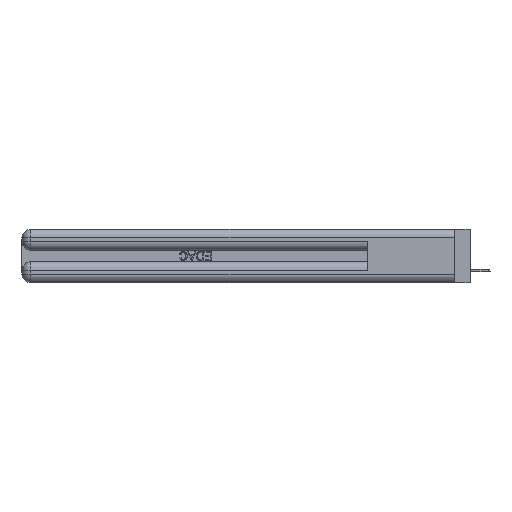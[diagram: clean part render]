
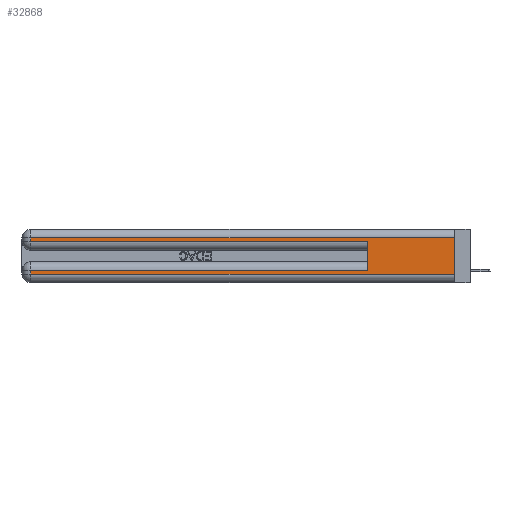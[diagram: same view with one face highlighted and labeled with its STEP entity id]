
A CAD part, left-side view. The second image highlights one B-rep face of the part: STEP entity #32868.
In plain terms, the highlighted planar face has unit normal (-1, 0, 0).
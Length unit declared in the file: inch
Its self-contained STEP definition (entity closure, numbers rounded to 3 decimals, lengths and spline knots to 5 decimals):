
#150 = LINE ( 'NONE', #11200, #28709 ) ;
#1371 = DIRECTION ( 'NONE',  ( 0., 0., -1. ) ) ;
#2030 = VECTOR ( 'NONE', #20193, 39.37008 ) ;
#3878 = VERTEX_POINT ( 'NONE', #27649 ) ;
#4669 = LINE ( 'NONE', #41682, #38491 ) ;
#5585 = LINE ( 'NONE', #27483, #32749 ) ;
#6645 = LINE ( 'NONE', #21100, #47113 ) ;
#8307 = DIRECTION ( 'NONE',  ( 0., 0., -1. ) ) ;
#8576 = PLANE ( 'NONE',  #41972 ) ;
#8738 = DIRECTION ( 'NONE',  ( 0., 0., -1. ) ) ;
#9347 = LINE ( 'NONE', #41319, #2030 ) ;
#10031 = EDGE_CURVE ( 'NONE', #31269, #13768, #5585, .T. ) ;
#10715 = VECTOR ( 'NONE', #8738, 39.37008 ) ;
#11078 = EDGE_CURVE ( 'NONE', #11703, #34523, #15241, .T. ) ;
#11200 = CARTESIAN_POINT ( 'NONE',  ( 0., 2.94, 0.37 ) ) ;
#11703 = VERTEX_POINT ( 'NONE', #31270 ) ;
#12193 = FACE_OUTER_BOUND ( 'NONE', #21809, .T. ) ;
#13702 = DIRECTION ( 'NONE',  ( 0., -1., 0. ) ) ;
#13768 = VERTEX_POINT ( 'NONE', #15794 ) ;
#15241 = LINE ( 'NONE', #32609, #22085 ) ;
#15722 = DIRECTION ( 'NONE',  ( 0., 1., 0. ) ) ;
#15794 = CARTESIAN_POINT ( 'NONE',  ( 0., 2.94, 0.06 ) ) ;
#15911 = ORIENTED_EDGE ( 'NONE', *, *, #23854, .T. ) ;
#17156 = ORIENTED_EDGE ( 'NONE', *, *, #30533, .F. ) ;
#18397 = EDGE_CURVE ( 'NONE', #34523, #3878, #150, .T. ) ;
#19479 = ORIENTED_EDGE ( 'NONE', *, *, #11078, .T. ) ;
#19950 = EDGE_CURVE ( 'NONE', #3878, #29705, #6645, .T. ) ;
#19963 = ORIENTED_EDGE ( 'NONE', *, *, #18397, .T. ) ;
#20193 = DIRECTION ( 'NONE',  ( 0., 1., 0. ) ) ;
#21100 = CARTESIAN_POINT ( 'NONE',  ( 0., 0., 0.285 ) ) ;
#21809 = EDGE_LOOP ( 'NONE', ( #17156, #19479, #19963, #46798, #38950, #22909, #43696, #15911 ) ) ;
#22085 = VECTOR ( 'NONE', #15722, 39.37008 ) ;
#22909 = ORIENTED_EDGE ( 'NONE', *, *, #34354, .T. ) ;
#23854 = EDGE_CURVE ( 'NONE', #13768, #40023, #25228, .T. ) ;
#25228 = LINE ( 'NONE', #28838, #31165 ) ;
#26618 = DIRECTION ( 'NONE',  ( 1., 0., 0. ) ) ;
#27032 = LINE ( 'NONE', #41670, #10715 ) ;
#27483 = CARTESIAN_POINT ( 'NONE',  ( 0., 2.94, 0.37 ) ) ;
#27649 = CARTESIAN_POINT ( 'NONE',  ( 0., 2.94, 0.285 ) ) ;
#28068 = DIRECTION ( 'NONE',  ( 0., -1., 0. ) ) ;
#28709 = VECTOR ( 'NONE', #8307, 39.37008 ) ;
#28838 = CARTESIAN_POINT ( 'NONE',  ( 0., 0., 0.06 ) ) ;
#29705 = VERTEX_POINT ( 'NONE', #42222 ) ;
#30533 = EDGE_CURVE ( 'NONE', #11703, #40023, #27032, .T. ) ;
#30535 = CARTESIAN_POINT ( 'NONE',  ( 0., 0.6, 0.085 ) ) ;
#31165 = VECTOR ( 'NONE', #13702, 39.37008 ) ;
#31269 = VERTEX_POINT ( 'NONE', #40127 ) ;
#31270 = CARTESIAN_POINT ( 'NONE',  ( 0., 0., 0.31 ) ) ;
#32609 = CARTESIAN_POINT ( 'NONE',  ( 0., 0., 0.31 ) ) ;
#32749 = VECTOR ( 'NONE', #42121, 39.37008 ) ;
#32868 = ADVANCED_FACE ( 'NONE', ( #12193 ), #8576, .F. ) ;
#34354 = EDGE_CURVE ( 'NONE', #35734, #31269, #9347, .T. ) ;
#34523 = VERTEX_POINT ( 'NONE', #38905 ) ;
#35734 = VERTEX_POINT ( 'NONE', #30535 ) ;
#37898 = CARTESIAN_POINT ( 'NONE',  ( 0., 0., 0.37 ) ) ;
#38073 = DIRECTION ( 'NONE',  ( 0., 0., 1. ) ) ;
#38491 = VECTOR ( 'NONE', #38073, 39.37008 ) ;
#38905 = CARTESIAN_POINT ( 'NONE',  ( 0., 2.94, 0.31 ) ) ;
#38950 = ORIENTED_EDGE ( 'NONE', *, *, #41998, .F. ) ;
#40023 = VERTEX_POINT ( 'NONE', #44696 ) ;
#40127 = CARTESIAN_POINT ( 'NONE',  ( 0., 2.94, 0.085 ) ) ;
#41319 = CARTESIAN_POINT ( 'NONE',  ( 0., 0., 0.085 ) ) ;
#41670 = CARTESIAN_POINT ( 'NONE',  ( 0., 0., 0.37 ) ) ;
#41682 = CARTESIAN_POINT ( 'NONE',  ( 0., 0.6, 0.145 ) ) ;
#41972 = AXIS2_PLACEMENT_3D ( 'NONE', #37898, #26618, #1371 ) ;
#41998 = EDGE_CURVE ( 'NONE', #35734, #29705, #4669, .T. ) ;
#42121 = DIRECTION ( 'NONE',  ( 0., 0., -1. ) ) ;
#42222 = CARTESIAN_POINT ( 'NONE',  ( 0., 0.6, 0.285 ) ) ;
#43696 = ORIENTED_EDGE ( 'NONE', *, *, #10031, .T. ) ;
#44696 = CARTESIAN_POINT ( 'NONE',  ( 0., 0., 0.06 ) ) ;
#46798 = ORIENTED_EDGE ( 'NONE', *, *, #19950, .T. ) ;
#47113 = VECTOR ( 'NONE', #28068, 39.37008 ) ;
